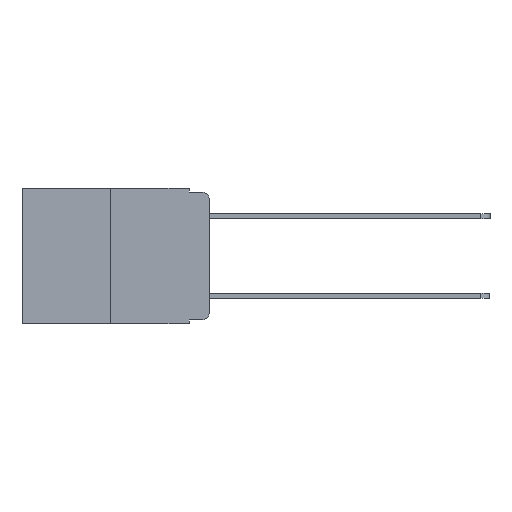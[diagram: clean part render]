
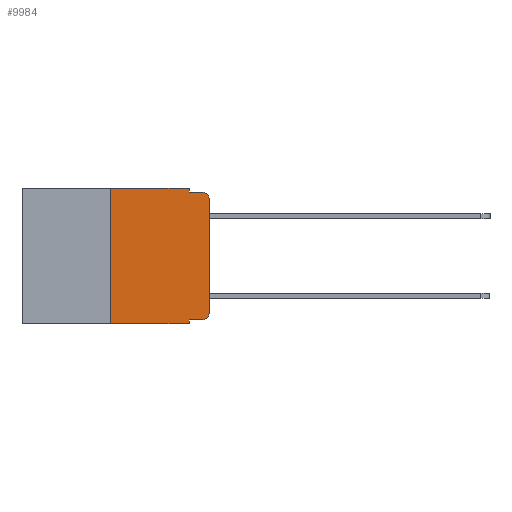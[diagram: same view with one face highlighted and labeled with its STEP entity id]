
A CAD part, left-side view. The second image highlights one B-rep face of the part: STEP entity #9984.
In plain terms, the highlighted planar face has unit normal (-1, 0, 0).
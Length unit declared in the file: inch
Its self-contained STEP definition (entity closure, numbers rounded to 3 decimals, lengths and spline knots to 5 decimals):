
#291 = CARTESIAN_POINT ( 'NONE',  ( 0., 0.25, 0. ) ) ;
#303 = VERTEX_POINT ( 'NONE', #1706 ) ;
#334 = EDGE_CURVE ( 'NONE', #8661, #1318, #5912, .T. ) ;
#394 = ORIENTED_EDGE ( 'NONE', *, *, #9343, .T. ) ;
#718 = VERTEX_POINT ( 'NONE', #4699 ) ;
#873 = DIRECTION ( 'NONE',  ( 0., -1., 0. ) ) ;
#976 = ORIENTED_EDGE ( 'NONE', *, *, #3760, .T. ) ;
#1050 = CARTESIAN_POINT ( 'NONE',  ( 0., 0.02, -0.313 ) ) ;
#1227 = VECTOR ( 'NONE', #2897, 39.37008 ) ;
#1318 = VERTEX_POINT ( 'NONE', #8114 ) ;
#1417 = VECTOR ( 'NONE', #6070, 39.37008 ) ;
#1544 = CARTESIAN_POINT ( 'NONE',  ( 0., 0.051, 0. ) ) ;
#1658 = PLANE ( 'NONE',  #1867 ) ;
#1706 = CARTESIAN_POINT ( 'NONE',  ( 0., 0., -0.313 ) ) ;
#1756 = VERTEX_POINT ( 'NONE', #10368 ) ;
#1867 = AXIS2_PLACEMENT_3D ( 'NONE', #11116, #9478, #4318 ) ;
#1916 = AXIS2_PLACEMENT_3D ( 'NONE', #1050, #7139, #1945 ) ;
#1945 = DIRECTION ( 'NONE',  ( 0., 0., -1. ) ) ;
#2120 = VERTEX_POINT ( 'NONE', #4683 ) ;
#2277 = CARTESIAN_POINT ( 'NONE',  ( 0., 0.473, 0. ) ) ;
#2897 = DIRECTION ( 'NONE',  ( 0., 0., 1. ) ) ;
#2989 = VECTOR ( 'NONE', #9427, 39.37008 ) ;
#3119 = ORIENTED_EDGE ( 'NONE', *, *, #4948, .F. ) ;
#3160 = CARTESIAN_POINT ( 'NONE',  ( 0., 0.051, -0.01 ) ) ;
#3597 = VERTEX_POINT ( 'NONE', #11157 ) ;
#3604 = EDGE_CURVE ( 'NONE', #8661, #8249, #10644, .T. ) ;
#3760 = EDGE_CURVE ( 'NONE', #303, #3597, #11283, .T. ) ;
#3769 = AXIS2_PLACEMENT_3D ( 'NONE', #9101, #3927, #9961 ) ;
#3927 = DIRECTION ( 'NONE',  ( -1., 0., 0. ) ) ;
#3995 = CARTESIAN_POINT ( 'NONE',  ( 0., 0.051, -0.01 ) ) ;
#4163 = CARTESIAN_POINT ( 'NONE',  ( 0., 0.25, -0.343 ) ) ;
#4181 = LINE ( 'NONE', #2277, #6215 ) ;
#4318 = DIRECTION ( 'NONE',  ( 0., 0., -1. ) ) ;
#4461 = VECTOR ( 'NONE', #10025, 39.37008 ) ;
#4488 = VECTOR ( 'NONE', #6385, 39.37008 ) ;
#4683 = CARTESIAN_POINT ( 'NONE',  ( 0., 0.051, -0.333 ) ) ;
#4699 = CARTESIAN_POINT ( 'NONE',  ( 0., 0.02, -0.333 ) ) ;
#4741 = VERTEX_POINT ( 'NONE', #7608 ) ;
#4743 = LINE ( 'NONE', #3995, #4461 ) ;
#4858 = EDGE_LOOP ( 'NONE', ( #976, #8596, #6588, #3119, #9225, #6488, #7998, #7016, #394, #5939 ) ) ;
#4948 = EDGE_CURVE ( 'NONE', #1756, #6402, #6077, .T. ) ;
#5542 = EDGE_CURVE ( 'NONE', #718, #303, #11243, .T. ) ;
#5912 = LINE ( 'NONE', #291, #1227 ) ;
#5939 = ORIENTED_EDGE ( 'NONE', *, *, #5542, .T. ) ;
#6070 = DIRECTION ( 'NONE',  ( 0., 0., -1. ) ) ;
#6077 = LINE ( 'NONE', #1544, #1417 ) ;
#6215 = VECTOR ( 'NONE', #6603, 39.37008 ) ;
#6379 = FACE_OUTER_BOUND ( 'NONE', #4858, .T. ) ;
#6385 = DIRECTION ( 'NONE',  ( 0., 0., 1. ) ) ;
#6402 = VERTEX_POINT ( 'NONE', #3160 ) ;
#6488 = ORIENTED_EDGE ( 'NONE', *, *, #334, .F. ) ;
#6588 = ORIENTED_EDGE ( 'NONE', *, *, #10921, .F. ) ;
#6603 = DIRECTION ( 'NONE',  ( 0., -1., 0. ) ) ;
#6606 = LINE ( 'NONE', #10409, #6866 ) ;
#6866 = VECTOR ( 'NONE', #11235, 39.37008 ) ;
#7016 = ORIENTED_EDGE ( 'NONE', *, *, #11123, .F. ) ;
#7139 = DIRECTION ( 'NONE',  ( -1., 0., 0. ) ) ;
#7608 = CARTESIAN_POINT ( 'NONE',  ( 0., 0.02, -0.01 ) ) ;
#7758 = CARTESIAN_POINT ( 'NONE',  ( 0., 0.473, -0.343 ) ) ;
#7998 = ORIENTED_EDGE ( 'NONE', *, *, #3604, .T. ) ;
#8114 = CARTESIAN_POINT ( 'NONE',  ( 0., 0.25, 0. ) ) ;
#8249 = VERTEX_POINT ( 'NONE', #9598 ) ;
#8472 = EDGE_CURVE ( 'NONE', #3597, #4741, #10419, .T. ) ;
#8527 = CARTESIAN_POINT ( 'NONE',  ( 0., 0.051, -0.333 ) ) ;
#8596 = ORIENTED_EDGE ( 'NONE', *, *, #8472, .T. ) ;
#8661 = VERTEX_POINT ( 'NONE', #4163 ) ;
#9101 = CARTESIAN_POINT ( 'NONE',  ( 0., 0.02, -0.03 ) ) ;
#9225 = ORIENTED_EDGE ( 'NONE', *, *, #10939, .F. ) ;
#9343 = EDGE_CURVE ( 'NONE', #2120, #718, #9872, .T. ) ;
#9414 = CARTESIAN_POINT ( 'NONE',  ( 0., 0., 0. ) ) ;
#9427 = DIRECTION ( 'NONE',  ( 0., -1., 0. ) ) ;
#9478 = DIRECTION ( 'NONE',  ( 1., 0., 0. ) ) ;
#9598 = CARTESIAN_POINT ( 'NONE',  ( 0., 0.051, -0.343 ) ) ;
#9872 = LINE ( 'NONE', #8527, #2989 ) ;
#9961 = DIRECTION ( 'NONE',  ( 0., 0., -1. ) ) ;
#9984 = ADVANCED_FACE ( 'NONE', ( #6379 ), #1658, .F. ) ;
#10025 = DIRECTION ( 'NONE',  ( 0., -1., 0. ) ) ;
#10368 = CARTESIAN_POINT ( 'NONE',  ( 0., 0.051, 0. ) ) ;
#10409 = CARTESIAN_POINT ( 'NONE',  ( 0., 0.051, 0. ) ) ;
#10419 = CIRCLE ( 'NONE', #3769, 0.02 ) ;
#10644 = LINE ( 'NONE', #7758, #10907 ) ;
#10907 = VECTOR ( 'NONE', #873, 39.37008 ) ;
#10921 = EDGE_CURVE ( 'NONE', #6402, #4741, #4743, .T. ) ;
#10939 = EDGE_CURVE ( 'NONE', #1318, #1756, #4181, .T. ) ;
#11116 = CARTESIAN_POINT ( 'NONE',  ( 0., 0.473, 0. ) ) ;
#11123 = EDGE_CURVE ( 'NONE', #2120, #8249, #6606, .T. ) ;
#11157 = CARTESIAN_POINT ( 'NONE',  ( 0., 0., -0.03 ) ) ;
#11235 = DIRECTION ( 'NONE',  ( 0., 0., -1. ) ) ;
#11243 = CIRCLE ( 'NONE', #1916, 0.02 ) ;
#11283 = LINE ( 'NONE', #9414, #4488 ) ;
